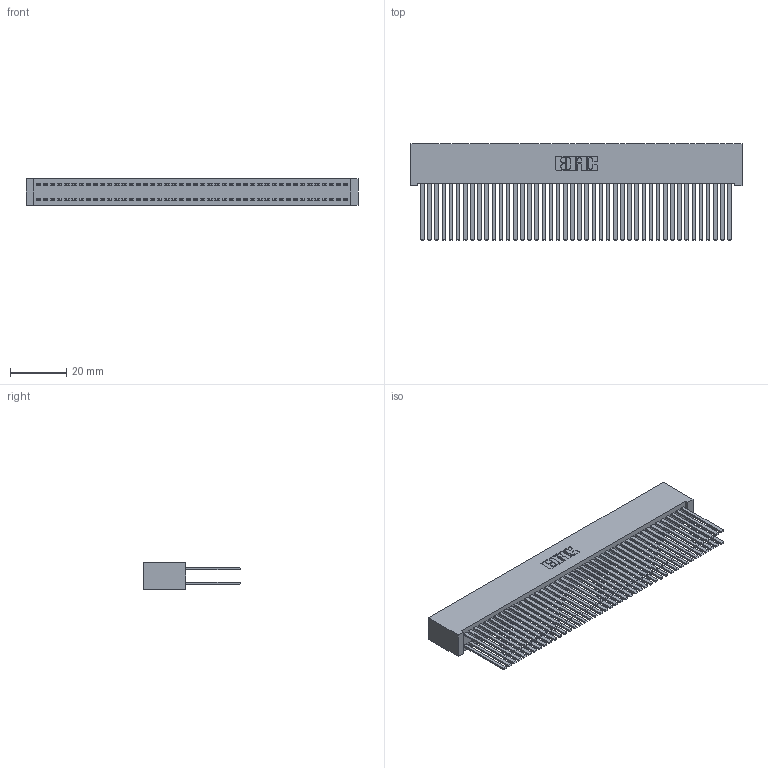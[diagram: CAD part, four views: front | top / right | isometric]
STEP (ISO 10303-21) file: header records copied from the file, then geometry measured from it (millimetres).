
FILE_DESCRIPTION (( 'STEP AP203' ), '1' );
FILE_NAME ('342-088-544-201.STEP', '2018-08-13T20:47:02', ( '' ), ( '' ), 'SwSTEP 2.0', 'SolidWorks 2016', '' );
FILE_SCHEMA (( 'CONFIG_CONTROL_DESIGN' ));
Length unit declared in the file: inch
Products named in the file (3): 342 Part_Lugless; 345-292-001_345-293-144; 342-088-544-201
Assembly tree (89 placements, depth 2):
  342-088-544-201
    342 Part_Lugless
    345-292-001_345-293-144  x88
Bounding box: 118.01 x 34.3 x 9.4 mm (x, y, z)
Volume: 12285.6 mm3; surface area: 23909.7 mm2
Topology: 89 solids, 89 shells, 4150 faces, 12331 edges, 8102 vertices
Faces by surface type: plane 2878, cylinder 1272
Entity records: 27455 total; most frequent: CARTESIAN_POINT 4542, ORIENTED_EDGE 4478, DIRECTION 3867, EDGE_CURVE 2239, VECTOR 2123, LINE 2123, VERTEX_POINT 1490, AXIS2_PLACEMENT_3D 872
